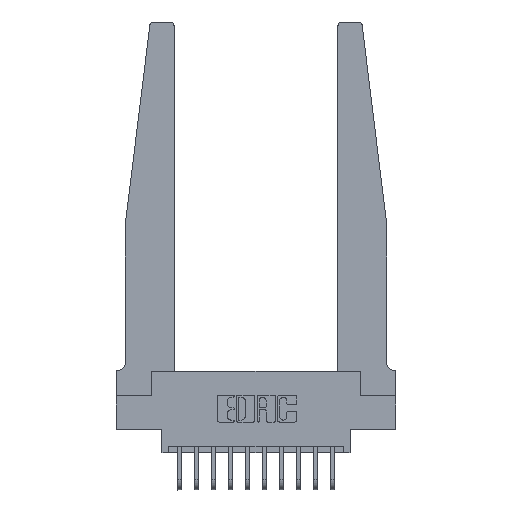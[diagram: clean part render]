
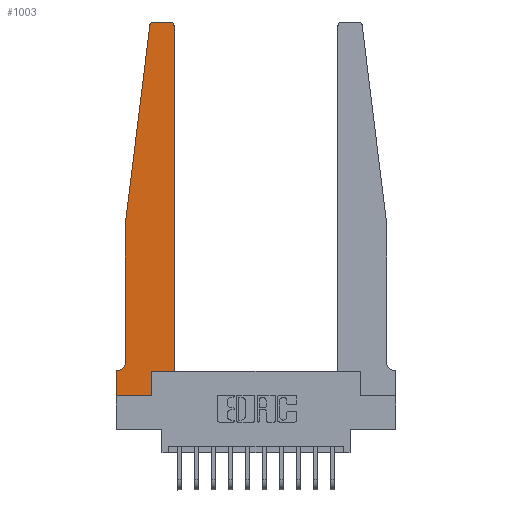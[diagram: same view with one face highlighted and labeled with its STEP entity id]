
A CAD part, top view. The second image highlights one B-rep face of the part: STEP entity #1003.
In plain terms, the highlighted planar face has unit normal (0, 0, 1).
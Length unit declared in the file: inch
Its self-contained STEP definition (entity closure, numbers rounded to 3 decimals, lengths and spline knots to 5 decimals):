
#211 = DIRECTION ( 'NONE',  ( -0.122, -0.992, 0. ) ) ;
#451 = CARTESIAN_POINT ( 'NONE',  ( 0.065, 1.25, 0.37 ) ) ;
#554 = CARTESIAN_POINT ( 'NONE',  ( 0.2605, 0., 0.37 ) ) ;
#754 = LINE ( 'NONE', #14994, #5017 ) ;
#977 = ORIENTED_EDGE ( 'NONE', *, *, #2389, .T. ) ;
#1003 = ADVANCED_FACE ( 'NONE', ( #7505 ), #5853, .T. ) ;
#1019 = CARTESIAN_POINT ( 'NONE',  ( 0.2605, 0.18, 0.37 ) ) ;
#1086 = VECTOR ( 'NONE', #8449, 39.37008 ) ;
#1318 = CARTESIAN_POINT ( 'NONE',  ( 0., 0., 0.37 ) ) ;
#1616 = ORIENTED_EDGE ( 'NONE', *, *, #11984, .T. ) ;
#1775 = CARTESIAN_POINT ( 'NONE',  ( 0.395, 2.72, 0.37 ) ) ;
#1850 = CIRCLE ( 'NONE', #13059, 0.05 ) ;
#1896 = AXIS2_PLACEMENT_3D ( 'NONE', #15321, #7231, #16922 ) ;
#2061 = DIRECTION ( 'NONE',  ( 1., 0., 0. ) ) ;
#2263 = ORIENTED_EDGE ( 'NONE', *, *, #12290, .T. ) ;
#2327 = DIRECTION ( 'NONE',  ( -1., 0., 0. ) ) ;
#2373 = DIRECTION ( 'NONE',  ( 0., 0., 1. ) ) ;
#2389 = EDGE_CURVE ( 'NONE', #15952, #13366, #14998, .T. ) ;
#2524 = LINE ( 'NONE', #1318, #10589 ) ;
#2526 = VECTOR ( 'NONE', #7143, 39.37008 ) ;
#2642 = EDGE_CURVE ( 'NONE', #8068, #5239, #7842, .T. ) ;
#2733 = CARTESIAN_POINT ( 'NONE',  ( 0.395, 2.75, 0.37 ) ) ;
#2782 = DIRECTION ( 'NONE',  ( 0., 0., -1. ) ) ;
#2872 = EDGE_CURVE ( 'NONE', #13366, #6291, #2524, .T. ) ;
#2931 = EDGE_CURVE ( 'NONE', #6401, #17057, #6785, .T. ) ;
#3318 = VERTEX_POINT ( 'NONE', #1019 ) ;
#3483 = EDGE_CURVE ( 'NONE', #5239, #6401, #12236, .T. ) ;
#3695 = CARTESIAN_POINT ( 'NONE',  ( 0.015, 0.1875, 0.37 ) ) ;
#3792 = VERTEX_POINT ( 'NONE', #9308 ) ;
#3794 = EDGE_CURVE ( 'NONE', #3792, #8068, #10326, .T. ) ;
#4057 = LINE ( 'NONE', #14518, #5963 ) ;
#4387 = CARTESIAN_POINT ( 'NONE',  ( 0.065, 0.1875, 0.37 ) ) ;
#4420 = ORIENTED_EDGE ( 'NONE', *, *, #17361, .T. ) ;
#4630 = ORIENTED_EDGE ( 'NONE', *, *, #2931, .T. ) ;
#4766 = AXIS2_PLACEMENT_3D ( 'NONE', #13162, #4987, #10419 ) ;
#4987 = DIRECTION ( 'NONE',  ( 0., 0., 1. ) ) ;
#5017 = VECTOR ( 'NONE', #10957, 39.37008 ) ;
#5239 = VERTEX_POINT ( 'NONE', #2733 ) ;
#5853 = PLANE ( 'NONE',  #1896 ) ;
#5866 = ORIENTED_EDGE ( 'NONE', *, *, #15377, .T. ) ;
#5963 = VECTOR ( 'NONE', #15886, 39.37008 ) ;
#6053 = CARTESIAN_POINT ( 'NONE',  ( 0.25, 2.75, 0.37 ) ) ;
#6291 = VERTEX_POINT ( 'NONE', #554 ) ;
#6401 = VERTEX_POINT ( 'NONE', #6639 ) ;
#6639 = CARTESIAN_POINT ( 'NONE',  ( 0.27653, 2.75, 0.37 ) ) ;
#6785 = CIRCLE ( 'NONE', #4766, 0.03 ) ;
#7028 = ORIENTED_EDGE ( 'NONE', *, *, #3794, .T. ) ;
#7143 = DIRECTION ( 'NONE',  ( 0., -1., 0. ) ) ;
#7231 = DIRECTION ( 'NONE',  ( 0., 0., 1. ) ) ;
#7268 = CARTESIAN_POINT ( 'NONE',  ( 0., 0., 0.37 ) ) ;
#7505 = FACE_OUTER_BOUND ( 'NONE', #16410, .T. ) ;
#7842 = CIRCLE ( 'NONE', #11084, 0.03 ) ;
#8011 = DIRECTION ( 'NONE',  ( 0., 1., 0. ) ) ;
#8068 = VERTEX_POINT ( 'NONE', #9162 ) ;
#8189 = CARTESIAN_POINT ( 'NONE',  ( 0.015, 0.2375, 0.37 ) ) ;
#8449 = DIRECTION ( 'NONE',  ( -1., 0., 0. ) ) ;
#8622 = EDGE_CURVE ( 'NONE', #3318, #3792, #13548, .T. ) ;
#9162 = CARTESIAN_POINT ( 'NONE',  ( 0.425, 2.72, 0.37 ) ) ;
#9308 = CARTESIAN_POINT ( 'NONE',  ( 0.425, 0.18, 0.37 ) ) ;
#9492 = VERTEX_POINT ( 'NONE', #13407 ) ;
#10153 = CARTESIAN_POINT ( 'NONE',  ( 0.065, 0.2375, 0.37 ) ) ;
#10326 = LINE ( 'NONE', #11974, #15403 ) ;
#10419 = DIRECTION ( 'NONE',  ( 1., 0., 0. ) ) ;
#10559 = VECTOR ( 'NONE', #2327, 39.37008 ) ;
#10589 = VECTOR ( 'NONE', #12145, 39.37008 ) ;
#10607 = DIRECTION ( 'NONE',  ( 1., 0., 0. ) ) ;
#10957 = DIRECTION ( 'NONE',  ( 0., 1., 0. ) ) ;
#11084 = AXIS2_PLACEMENT_3D ( 'NONE', #1775, #2373, #10607 ) ;
#11560 = LINE ( 'NONE', #451, #12618 ) ;
#11591 = CARTESIAN_POINT ( 'NONE',  ( 0.425, 0.18, 0.37 ) ) ;
#11841 = ORIENTED_EDGE ( 'NONE', *, *, #8622, .T. ) ;
#11904 = VERTEX_POINT ( 'NONE', #10153 ) ;
#11974 = CARTESIAN_POINT ( 'NONE',  ( 0.425, 0.18, 0.37 ) ) ;
#11984 = EDGE_CURVE ( 'NONE', #9492, #11904, #4057, .T. ) ;
#12145 = DIRECTION ( 'NONE',  ( 1., 0., 0. ) ) ;
#12151 = CARTESIAN_POINT ( 'NONE',  ( 0.24675, 2.72367, 0.37 ) ) ;
#12236 = LINE ( 'NONE', #6053, #10559 ) ;
#12251 = DIRECTION ( 'NONE',  ( -1., 0., 0. ) ) ;
#12290 = EDGE_CURVE ( 'NONE', #13478, #15952, #15281, .T. ) ;
#12618 = VECTOR ( 'NONE', #211, 39.37008 ) ;
#13053 = ORIENTED_EDGE ( 'NONE', *, *, #2872, .T. ) ;
#13059 = AXIS2_PLACEMENT_3D ( 'NONE', #8189, #2782, #12251 ) ;
#13162 = CARTESIAN_POINT ( 'NONE',  ( 0.27653, 2.72, 0.37 ) ) ;
#13366 = VERTEX_POINT ( 'NONE', #7268 ) ;
#13407 = CARTESIAN_POINT ( 'NONE',  ( 0.065, 1.25, 0.37 ) ) ;
#13478 = VERTEX_POINT ( 'NONE', #3695 ) ;
#13548 = LINE ( 'NONE', #11591, #16727 ) ;
#13763 = CARTESIAN_POINT ( 'NONE',  ( 0., 0.1875, 0.37 ) ) ;
#13894 = ORIENTED_EDGE ( 'NONE', *, *, #15610, .T. ) ;
#14518 = CARTESIAN_POINT ( 'NONE',  ( 0.065, 1.25, 0.37 ) ) ;
#14994 = CARTESIAN_POINT ( 'NONE',  ( 0.2605, 0.18, 0.37 ) ) ;
#14998 = LINE ( 'NONE', #15232, #2526 ) ;
#15232 = CARTESIAN_POINT ( 'NONE',  ( 0., 0., 0.37 ) ) ;
#15281 = LINE ( 'NONE', #4387, #1086 ) ;
#15321 = CARTESIAN_POINT ( 'NONE',  ( 0., 0.1875, 0.37 ) ) ;
#15377 = EDGE_CURVE ( 'NONE', #6291, #3318, #754, .T. ) ;
#15403 = VECTOR ( 'NONE', #8011, 39.37008 ) ;
#15610 = EDGE_CURVE ( 'NONE', #17057, #9492, #11560, .T. ) ;
#15886 = DIRECTION ( 'NONE',  ( 0., -1., 0. ) ) ;
#15952 = VERTEX_POINT ( 'NONE', #13763 ) ;
#16410 = EDGE_LOOP ( 'NONE', ( #16566, #4630, #13894, #1616, #4420, #2263, #977, #13053, #5866, #11841, #7028, #16584 ) ) ;
#16566 = ORIENTED_EDGE ( 'NONE', *, *, #3483, .T. ) ;
#16584 = ORIENTED_EDGE ( 'NONE', *, *, #2642, .T. ) ;
#16727 = VECTOR ( 'NONE', #2061, 39.37008 ) ;
#16922 = DIRECTION ( 'NONE',  ( 1., 0., 0. ) ) ;
#17057 = VERTEX_POINT ( 'NONE', #12151 ) ;
#17361 = EDGE_CURVE ( 'NONE', #11904, #13478, #1850, .T. ) ;
